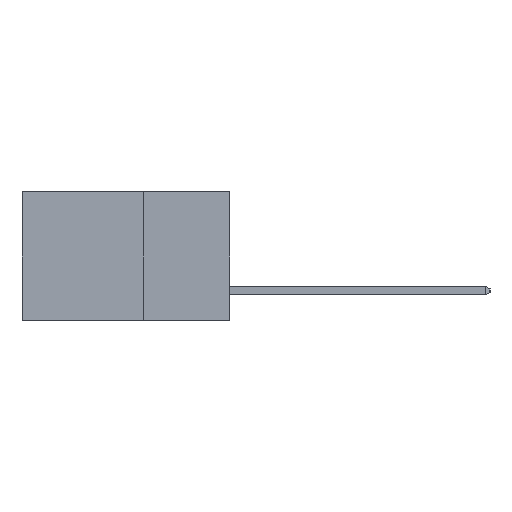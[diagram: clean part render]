
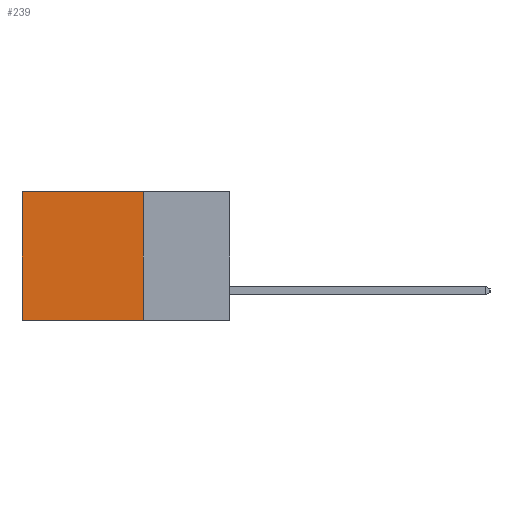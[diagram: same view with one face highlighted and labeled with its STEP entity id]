
A CAD part, left-side view. The second image highlights one B-rep face of the part: STEP entity #239.
In plain terms, the highlighted planar face has unit normal (-1, 0, 0).
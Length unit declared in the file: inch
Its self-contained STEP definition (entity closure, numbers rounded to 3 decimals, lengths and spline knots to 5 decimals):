
#150 = EDGE_CURVE ( 'NONE', #9552, #10083, #4505, .T. ) ;
#239 = ADVANCED_FACE ( 'NONE', ( #10802 ), #12286, .F. ) ;
#1472 = VECTOR ( 'NONE', #1594, 39.37008 ) ;
#1594 = DIRECTION ( 'NONE',  ( 0., 0., -1. ) ) ;
#1664 = CARTESIAN_POINT ( 'NONE',  ( 0.2615, 0.6, 0. ) ) ;
#2138 = CARTESIAN_POINT ( 'NONE',  ( 0.2615, 0.25, 0. ) ) ;
#2152 = CARTESIAN_POINT ( 'NONE',  ( 0.2615, 0.6, -0.37 ) ) ;
#3294 = CARTESIAN_POINT ( 'NONE',  ( 0.2615, 0.25, 0. ) ) ;
#3828 = CARTESIAN_POINT ( 'NONE',  ( 0.2615, 0.25, -0.37 ) ) ;
#4395 = VERTEX_POINT ( 'NONE', #3294 ) ;
#4505 = LINE ( 'NONE', #2152, #1472 ) ;
#4714 = ORIENTED_EDGE ( 'NONE', *, *, #8956, .F. ) ;
#4837 = VECTOR ( 'NONE', #11746, 39.37008 ) ;
#5318 = EDGE_LOOP ( 'NONE', ( #6098, #12241, #4714, #8842 ) ) ;
#6098 = ORIENTED_EDGE ( 'NONE', *, *, #150, .T. ) ;
#6750 = EDGE_CURVE ( 'NONE', #12708, #10083, #9047, .T. ) ;
#7244 = LINE ( 'NONE', #2138, #7563 ) ;
#7563 = VECTOR ( 'NONE', #10387, 39.37008 ) ;
#7574 = LINE ( 'NONE', #7582, #4837 ) ;
#7582 = CARTESIAN_POINT ( 'NONE',  ( 0.2615, 0.25, -0.37 ) ) ;
#8731 = VECTOR ( 'NONE', #9938, 39.37008 ) ;
#8842 = ORIENTED_EDGE ( 'NONE', *, *, #9282, .T. ) ;
#8956 = EDGE_CURVE ( 'NONE', #4395, #12708, #7574, .T. ) ;
#9047 = LINE ( 'NONE', #3828, #8731 ) ;
#9282 = EDGE_CURVE ( 'NONE', #4395, #9552, #7244, .T. ) ;
#9552 = VERTEX_POINT ( 'NONE', #1664 ) ;
#9569 = AXIS2_PLACEMENT_3D ( 'NONE', #12207, #12238, #12164 ) ;
#9938 = DIRECTION ( 'NONE',  ( 0., 1., 0. ) ) ;
#10083 = VERTEX_POINT ( 'NONE', #10963 ) ;
#10295 = CARTESIAN_POINT ( 'NONE',  ( 0.2615, 0.25, -0.37 ) ) ;
#10387 = DIRECTION ( 'NONE',  ( 0., 1., 0. ) ) ;
#10802 = FACE_OUTER_BOUND ( 'NONE', #5318, .T. ) ;
#10963 = CARTESIAN_POINT ( 'NONE',  ( 0.2615, 0.6, -0.37 ) ) ;
#11746 = DIRECTION ( 'NONE',  ( 0., 0., -1. ) ) ;
#12164 = DIRECTION ( 'NONE',  ( 0., 0., -1. ) ) ;
#12207 = CARTESIAN_POINT ( 'NONE',  ( 0.2615, 0.25, -0.37 ) ) ;
#12238 = DIRECTION ( 'NONE',  ( 1., 0., 0. ) ) ;
#12241 = ORIENTED_EDGE ( 'NONE', *, *, #6750, .F. ) ;
#12286 = PLANE ( 'NONE',  #9569 ) ;
#12708 = VERTEX_POINT ( 'NONE', #10295 ) ;
